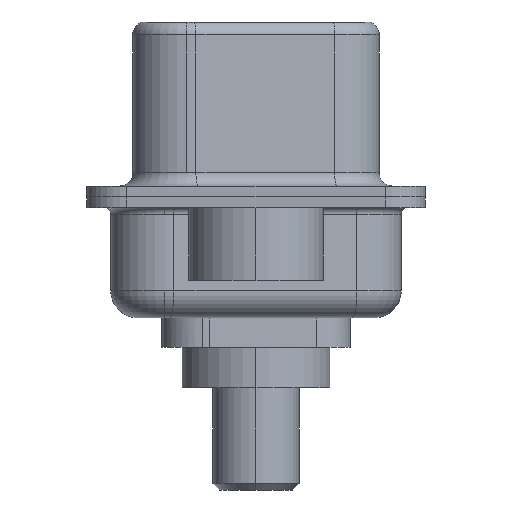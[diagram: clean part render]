
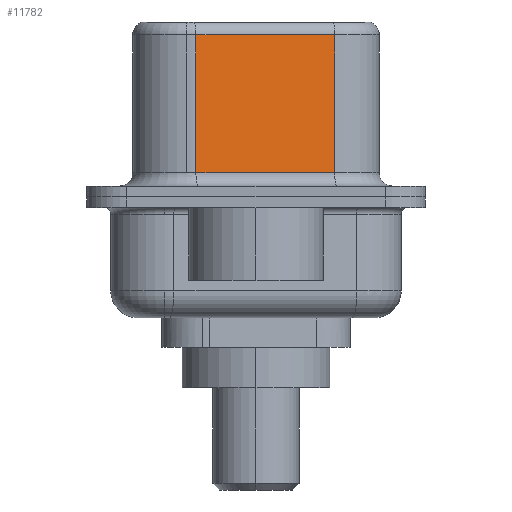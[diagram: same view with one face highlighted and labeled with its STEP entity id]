
A CAD part, left-side view. The second image highlights one B-rep face of the part: STEP entity #11782.
In plain terms, the highlighted planar face has unit normal (-0.985, -0.174, 0).
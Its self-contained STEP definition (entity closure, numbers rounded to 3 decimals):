
#49 = FACE_OUTER_BOUND ( 'NONE', #4026, .T. ) ;
#180 = VECTOR ( 'NONE', #10762, 1000. ) ;
#435 = DIRECTION ( 'NONE',  ( -0.174, 0.985, 0. ) ) ;
#648 = EDGE_CURVE ( 'NONE', #4063, #11594, #9110, .T. ) ;
#870 = CARTESIAN_POINT ( 'NONE',  ( 3.67, 2.233, 6.52 ) ) ;
#1006 = ORIENTED_EDGE ( 'NONE', *, *, #648, .T. ) ;
#1460 = PLANE ( 'NONE',  #12471 ) ;
#2630 = ORIENTED_EDGE ( 'NONE', *, *, #6298, .T. ) ;
#3158 = VECTOR ( 'NONE', #7695, 1000. ) ;
#3827 = CARTESIAN_POINT ( 'NONE',  ( 4.58, -2.927, 6.02 ) ) ;
#4026 = EDGE_LOOP ( 'NONE', ( #4845, #1006, #2630, #12331 ) ) ;
#4063 = VERTEX_POINT ( 'NONE', #10336 ) ;
#4653 = LINE ( 'NONE', #870, #7657 ) ;
#4845 = ORIENTED_EDGE ( 'NONE', *, *, #5564, .F. ) ;
#5488 = VERTEX_POINT ( 'NONE', #13873 ) ;
#5564 = EDGE_CURVE ( 'NONE', #4063, #5488, #6070, .T. ) ;
#5948 = CARTESIAN_POINT ( 'NONE',  ( 4.58, -2.927, 6.52 ) ) ;
#6070 = LINE ( 'NONE', #11839, #180 ) ;
#6134 = LINE ( 'NONE', #11932, #3158 ) ;
#6298 = EDGE_CURVE ( 'NONE', #11594, #12836, #4653, .T. ) ;
#7100 = DIRECTION ( 'NONE',  ( 0.985, 0.174, 0. ) ) ;
#7657 = VECTOR ( 'NONE', #8676, 1000. ) ;
#7695 = DIRECTION ( 'NONE',  ( 0.174, -0.985, 0. ) ) ;
#8676 = DIRECTION ( 'NONE',  ( 0., 0., -1. ) ) ;
#9110 = LINE ( 'NONE', #3827, #11912 ) ;
#10003 = CARTESIAN_POINT ( 'NONE',  ( 3.67, 2.233, 6.02 ) ) ;
#10336 = CARTESIAN_POINT ( 'NONE',  ( 4.58, -2.927, 6.02 ) ) ;
#10693 = DIRECTION ( 'NONE',  ( -0.174, 0.985, 0. ) ) ;
#10762 = DIRECTION ( 'NONE',  ( 0., 0., -1. ) ) ;
#11420 = EDGE_CURVE ( 'NONE', #12836, #5488, #6134, .T. ) ;
#11594 = VERTEX_POINT ( 'NONE', #10003 ) ;
#11782 = ADVANCED_FACE ( 'NONE', ( #49 ), #1460, .F. ) ;
#11839 = CARTESIAN_POINT ( 'NONE',  ( 4.58, -2.927, 6.52 ) ) ;
#11912 = VECTOR ( 'NONE', #10693, 1000. ) ;
#11932 = CARTESIAN_POINT ( 'NONE',  ( 4.58, -2.927, 0.9 ) ) ;
#12331 = ORIENTED_EDGE ( 'NONE', *, *, #11420, .T. ) ;
#12471 = AXIS2_PLACEMENT_3D ( 'NONE', #5948, #7100, #435 ) ;
#12836 = VERTEX_POINT ( 'NONE', #13309 ) ;
#13309 = CARTESIAN_POINT ( 'NONE',  ( 3.67, 2.233, 0.9 ) ) ;
#13873 = CARTESIAN_POINT ( 'NONE',  ( 4.58, -2.927, 0.9 ) ) ;
